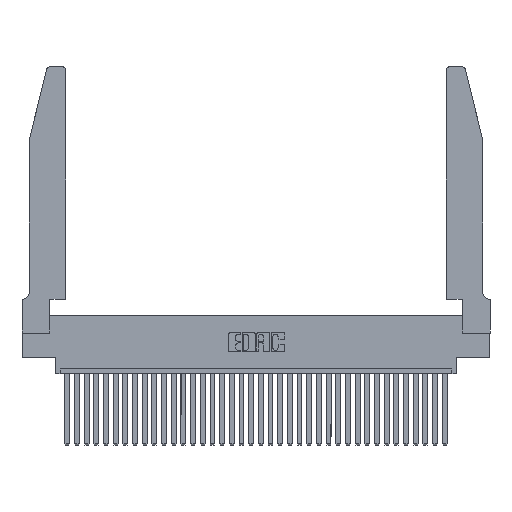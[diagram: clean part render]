
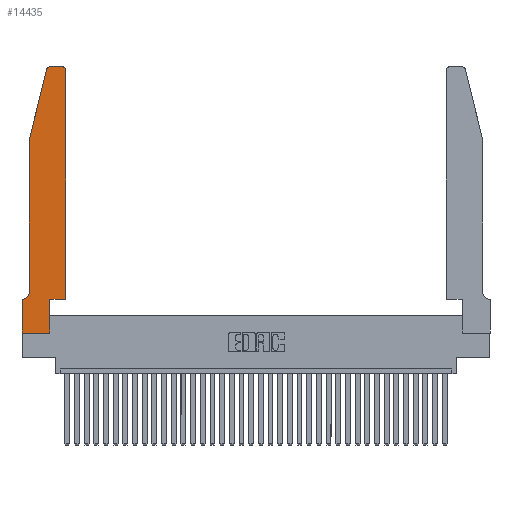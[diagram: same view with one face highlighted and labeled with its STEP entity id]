
A CAD part, top view. The second image highlights one B-rep face of the part: STEP entity #14435.
In plain terms, the highlighted planar face has unit normal (0, 0, 1).
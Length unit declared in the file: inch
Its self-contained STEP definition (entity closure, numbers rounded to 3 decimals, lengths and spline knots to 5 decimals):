
#310 = CARTESIAN_POINT ( 'NONE',  ( 0.4505, 0.35, 0.37 ) ) ;
#809 = ORIENTED_EDGE ( 'NONE', *, *, #30172, .T. ) ;
#929 = VECTOR ( 'NONE', #35089, 39.37008 ) ;
#980 = CARTESIAN_POINT ( 'NONE',  ( 0.4505, 0.35, 0.37 ) ) ;
#1035 = VERTEX_POINT ( 'NONE', #22514 ) ;
#1070 = CARTESIAN_POINT ( 'NONE',  ( 0., 0.35, 0.37 ) ) ;
#1104 = DIRECTION ( 'NONE',  ( 1., 0., 0. ) ) ;
#1152 = EDGE_CURVE ( 'NONE', #17943, #25825, #34804, .T. ) ;
#1946 = EDGE_CURVE ( 'NONE', #22063, #15057, #2196, .T. ) ;
#2196 = CIRCLE ( 'NONE', #21957, 0.03 ) ;
#3231 = CARTESIAN_POINT ( 'NONE',  ( 0., 0., 0.37 ) ) ;
#3412 = CARTESIAN_POINT ( 'NONE',  ( 0., 0.35, 0.37 ) ) ;
#4220 = DIRECTION ( 'NONE',  ( 0., -1., 0. ) ) ;
#4693 = ORIENTED_EDGE ( 'NONE', *, *, #30970, .T. ) ;
#5448 = LINE ( 'NONE', #310, #30363 ) ;
#6182 = DIRECTION ( 'NONE',  ( 1., 0., 0. ) ) ;
#6462 = CARTESIAN_POINT ( 'NONE',  ( 0.0755, 2., 0.37 ) ) ;
#6642 = DIRECTION ( 'NONE',  ( -1., 0., 0. ) ) ;
#6738 = EDGE_CURVE ( 'NONE', #25825, #18197, #17848, .T. ) ;
#7141 = FACE_OUTER_BOUND ( 'NONE', #27450, .T. ) ;
#7163 = CIRCLE ( 'NONE', #31384, 0.03 ) ;
#8349 = EDGE_CURVE ( 'NONE', #18197, #35004, #8417, .T. ) ;
#8417 = LINE ( 'NONE', #30717, #29150 ) ;
#8670 = CARTESIAN_POINT ( 'NONE',  ( 0.284, 2.75, 0.37 ) ) ;
#8762 = CARTESIAN_POINT ( 'NONE',  ( 0.0755, 0.35, 0.37 ) ) ;
#8801 = CARTESIAN_POINT ( 'NONE',  ( 0.0755, 2., 0.37 ) ) ;
#8870 = VERTEX_POINT ( 'NONE', #18195 ) ;
#9051 = DIRECTION ( 'NONE',  ( -0.239, -0.971, 0. ) ) ;
#9513 = VERTEX_POINT ( 'NONE', #23013 ) ;
#10491 = LINE ( 'NONE', #22686, #34178 ) ;
#10779 = EDGE_CURVE ( 'NONE', #11186, #9513, #25161, .T. ) ;
#10803 = VECTOR ( 'NONE', #34082, 39.37008 ) ;
#11186 = VERTEX_POINT ( 'NONE', #6462 ) ;
#11483 = DIRECTION ( 'NONE',  ( 0., 0., 1. ) ) ;
#12205 = AXIS2_PLACEMENT_3D ( 'NONE', #1070, #30623, #6182 ) ;
#12620 = LINE ( 'NONE', #980, #25721 ) ;
#13016 = EDGE_CURVE ( 'NONE', #9513, #8870, #17345, .T. ) ;
#13147 = ORIENTED_EDGE ( 'NONE', *, *, #13877, .T. ) ;
#13877 = EDGE_CURVE ( 'NONE', #24748, #11186, #29929, .T. ) ;
#13941 = VERTEX_POINT ( 'NONE', #8670 ) ;
#14172 = ORIENTED_EDGE ( 'NONE', *, *, #8349, .T. ) ;
#14244 = CARTESIAN_POINT ( 'NONE',  ( 0.4205, 2.75, 0.37 ) ) ;
#14435 = ADVANCED_FACE ( 'NONE', ( #7141 ), #25314, .T. ) ;
#14473 = DIRECTION ( 'NONE',  ( -1., 0., 0. ) ) ;
#14824 = CARTESIAN_POINT ( 'NONE',  ( 0., 0., 0.37 ) ) ;
#15057 = VERTEX_POINT ( 'NONE', #14244 ) ;
#15893 = CARTESIAN_POINT ( 'NONE',  ( 0.2865, 0.35, 0.37 ) ) ;
#16817 = CARTESIAN_POINT ( 'NONE',  ( 0.2865, 0., 0.37 ) ) ;
#17043 = CARTESIAN_POINT ( 'NONE',  ( 0.4205, 2.72, 0.37 ) ) ;
#17272 = DIRECTION ( 'NONE',  ( 0., 0., 1. ) ) ;
#17345 = CIRCLE ( 'NONE', #21427, 0.07 ) ;
#17848 = LINE ( 'NONE', #23964, #929 ) ;
#17943 = VERTEX_POINT ( 'NONE', #3412 ) ;
#18157 = CARTESIAN_POINT ( 'NONE',  ( 0.25487, 2.72718, 0.37 ) ) ;
#18195 = CARTESIAN_POINT ( 'NONE',  ( 0.0055, 0.35, 0.37 ) ) ;
#18197 = VERTEX_POINT ( 'NONE', #16817 ) ;
#19479 = ORIENTED_EDGE ( 'NONE', *, *, #6738, .T. ) ;
#19705 = ORIENTED_EDGE ( 'NONE', *, *, #10779, .T. ) ;
#20129 = CARTESIAN_POINT ( 'NONE',  ( 0.4505, 2.72, 0.37 ) ) ;
#20453 = EDGE_CURVE ( 'NONE', #13941, #24748, #7163, .T. ) ;
#20592 = DIRECTION ( 'NONE',  ( 1., 0., 0. ) ) ;
#20787 = CARTESIAN_POINT ( 'NONE',  ( 0.0755, 2., 0.37 ) ) ;
#20943 = ORIENTED_EDGE ( 'NONE', *, *, #1946, .T. ) ;
#20978 = EDGE_CURVE ( 'NONE', #35004, #1035, #12620, .T. ) ;
#21250 = EDGE_CURVE ( 'NONE', #8870, #17943, #29856, .T. ) ;
#21427 = AXIS2_PLACEMENT_3D ( 'NONE', #22535, #22247, #14473 ) ;
#21596 = DIRECTION ( 'NONE',  ( 0., 1., 0. ) ) ;
#21957 = AXIS2_PLACEMENT_3D ( 'NONE', #17043, #17272, #1104 ) ;
#22063 = VERTEX_POINT ( 'NONE', #20129 ) ;
#22247 = DIRECTION ( 'NONE',  ( 0., 0., -1. ) ) ;
#22372 = VECTOR ( 'NONE', #9051, 39.37008 ) ;
#22514 = CARTESIAN_POINT ( 'NONE',  ( 0.4505, 0.35, 0.37 ) ) ;
#22535 = CARTESIAN_POINT ( 'NONE',  ( 0.0055, 0.42, 0.37 ) ) ;
#22686 = CARTESIAN_POINT ( 'NONE',  ( 0.2605, 2.75, 0.37 ) ) ;
#22720 = DIRECTION ( 'NONE',  ( -1., 0., 0. ) ) ;
#23013 = CARTESIAN_POINT ( 'NONE',  ( 0.0755, 0.42, 0.37 ) ) ;
#23618 = VECTOR ( 'NONE', #22720, 39.37008 ) ;
#23964 = CARTESIAN_POINT ( 'NONE',  ( 0., 0., 0.37 ) ) ;
#24413 = ORIENTED_EDGE ( 'NONE', *, *, #20453, .T. ) ;
#24748 = VERTEX_POINT ( 'NONE', #18157 ) ;
#25161 = LINE ( 'NONE', #20787, #10803 ) ;
#25314 = PLANE ( 'NONE',  #12205 ) ;
#25721 = VECTOR ( 'NONE', #20592, 39.37008 ) ;
#25825 = VERTEX_POINT ( 'NONE', #3231 ) ;
#25975 = ORIENTED_EDGE ( 'NONE', *, *, #21250, .T. ) ;
#27450 = EDGE_LOOP ( 'NONE', ( #4693, #24413, #13147, #19705, #32487, #25975, #29378, #19479, #14172, #30059, #809, #20943 ) ) ;
#27623 = CARTESIAN_POINT ( 'NONE',  ( 0.284, 2.72, 0.37 ) ) ;
#29150 = VECTOR ( 'NONE', #30837, 39.37008 ) ;
#29378 = ORIENTED_EDGE ( 'NONE', *, *, #1152, .T. ) ;
#29856 = LINE ( 'NONE', #8762, #23618 ) ;
#29929 = LINE ( 'NONE', #8801, #22372 ) ;
#30059 = ORIENTED_EDGE ( 'NONE', *, *, #20978, .T. ) ;
#30105 = VECTOR ( 'NONE', #4220, 39.37008 ) ;
#30172 = EDGE_CURVE ( 'NONE', #1035, #22063, #5448, .T. ) ;
#30358 = DIRECTION ( 'NONE',  ( 1., 0., 0. ) ) ;
#30363 = VECTOR ( 'NONE', #21596, 39.37008 ) ;
#30623 = DIRECTION ( 'NONE',  ( 0., 0., 1. ) ) ;
#30717 = CARTESIAN_POINT ( 'NONE',  ( 0.2865, 0.35, 0.37 ) ) ;
#30837 = DIRECTION ( 'NONE',  ( 0., 1., 0. ) ) ;
#30970 = EDGE_CURVE ( 'NONE', #15057, #13941, #10491, .T. ) ;
#31384 = AXIS2_PLACEMENT_3D ( 'NONE', #27623, #11483, #30358 ) ;
#32487 = ORIENTED_EDGE ( 'NONE', *, *, #13016, .T. ) ;
#34082 = DIRECTION ( 'NONE',  ( 0., -1., 0. ) ) ;
#34178 = VECTOR ( 'NONE', #6642, 39.37008 ) ;
#34804 = LINE ( 'NONE', #14824, #30105 ) ;
#35004 = VERTEX_POINT ( 'NONE', #15893 ) ;
#35089 = DIRECTION ( 'NONE',  ( 1., 0., 0. ) ) ;
